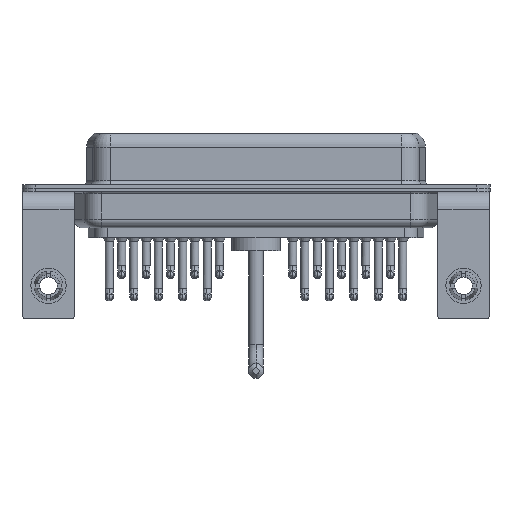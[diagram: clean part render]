
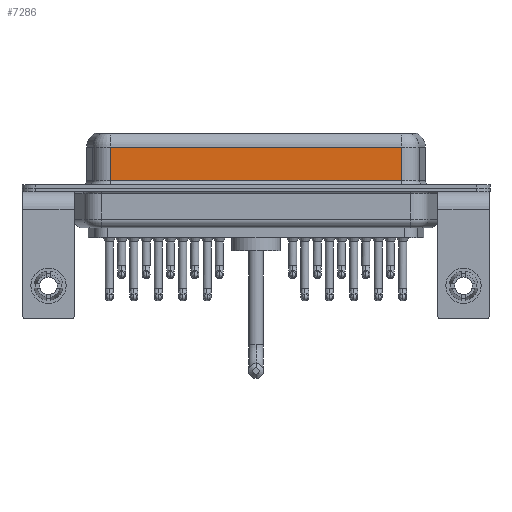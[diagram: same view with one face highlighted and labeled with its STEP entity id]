
A CAD part, front view. The second image highlights one B-rep face of the part: STEP entity #7286.
In plain terms, the highlighted planar face has unit normal (0, -1, 0).
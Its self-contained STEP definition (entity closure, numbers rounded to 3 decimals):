
#449 = EDGE_CURVE ( 'NONE', #19844, #22812, #11446, .T. ) ;
#1607 = CARTESIAN_POINT ( 'NONE',  ( 7.013, -3.95, 6.4 ) ) ;
#3114 = AXIS2_PLACEMENT_3D ( 'NONE', #14122, #17796, #4490 ) ;
#3221 = EDGE_CURVE ( 'NONE', #23335, #22101, #16667, .T. ) ;
#3363 = EDGE_CURVE ( 'NONE', #19844, #22101, #9566, .T. ) ;
#3753 = EDGE_CURVE ( 'NONE', #22812, #23335, #22878, .T. ) ;
#4490 = DIRECTION ( 'NONE',  ( 0., 0., 1. ) ) ;
#4649 = CARTESIAN_POINT ( 'NONE',  ( 40.037, -3.95, 0.9 ) ) ;
#7286 = ADVANCED_FACE ( 'NONE', ( #21994 ), #19711, .F. ) ;
#7311 = DIRECTION ( 'NONE',  ( 0., 0., -1. ) ) ;
#7683 = CARTESIAN_POINT ( 'NONE',  ( 40.037, -3.95, 4.65 ) ) ;
#8567 = DIRECTION ( 'NONE',  ( 1., 0., 0. ) ) ;
#9000 = VECTOR ( 'NONE', #23019, 1000. ) ;
#9436 = CARTESIAN_POINT ( 'NONE',  ( 40.037, -3.95, 6.4 ) ) ;
#9566 = LINE ( 'NONE', #9436, #9783 ) ;
#9746 = ORIENTED_EDGE ( 'NONE', *, *, #3363, .F. ) ;
#9783 = VECTOR ( 'NONE', #7311, 1000. ) ;
#11446 = LINE ( 'NONE', #7683, #23093 ) ;
#13122 = ORIENTED_EDGE ( 'NONE', *, *, #3221, .T. ) ;
#13532 = CARTESIAN_POINT ( 'NONE',  ( 7.013, -3.95, 4.65 ) ) ;
#14122 = CARTESIAN_POINT ( 'NONE',  ( 40.037, -3.95, 6.4 ) ) ;
#15463 = EDGE_LOOP ( 'NONE', ( #9746, #18337, #19509, #13122 ) ) ;
#16667 = LINE ( 'NONE', #4649, #18297 ) ;
#17796 = DIRECTION ( 'NONE',  ( 0., 1., 0. ) ) ;
#18297 = VECTOR ( 'NONE', #8567, 1000. ) ;
#18337 = ORIENTED_EDGE ( 'NONE', *, *, #449, .T. ) ;
#19091 = DIRECTION ( 'NONE',  ( -1., 0., 0. ) ) ;
#19509 = ORIENTED_EDGE ( 'NONE', *, *, #3753, .T. ) ;
#19711 = PLANE ( 'NONE',  #3114 ) ;
#19844 = VERTEX_POINT ( 'NONE', #21877 ) ;
#20126 = CARTESIAN_POINT ( 'NONE',  ( 7.013, -3.95, 0.9 ) ) ;
#20335 = CARTESIAN_POINT ( 'NONE',  ( 40.037, -3.95, 0.9 ) ) ;
#21877 = CARTESIAN_POINT ( 'NONE',  ( 40.037, -3.95, 4.65 ) ) ;
#21994 = FACE_OUTER_BOUND ( 'NONE', #15463, .T. ) ;
#22101 = VERTEX_POINT ( 'NONE', #20335 ) ;
#22812 = VERTEX_POINT ( 'NONE', #13532 ) ;
#22878 = LINE ( 'NONE', #1607, #9000 ) ;
#23019 = DIRECTION ( 'NONE',  ( 0., 0., -1. ) ) ;
#23093 = VECTOR ( 'NONE', #19091, 1000. ) ;
#23335 = VERTEX_POINT ( 'NONE', #20126 ) ;
